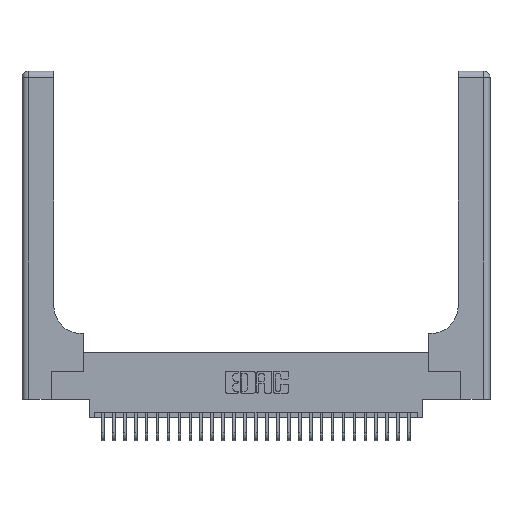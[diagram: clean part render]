
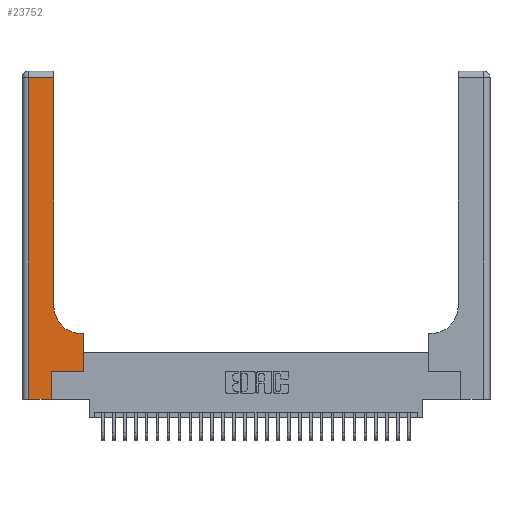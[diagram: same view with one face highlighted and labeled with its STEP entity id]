
A CAD part, top view. The second image highlights one B-rep face of the part: STEP entity #23752.
In plain terms, the highlighted planar face has unit normal (0, 0, 1).
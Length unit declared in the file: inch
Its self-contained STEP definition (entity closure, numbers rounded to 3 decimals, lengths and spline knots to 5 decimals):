
#189 = LINE ( 'NONE', #30230, #536 ) ;
#536 = VECTOR ( 'NONE', #6259, 39.37008 ) ;
#762 = VERTEX_POINT ( 'NONE', #8528 ) ;
#2404 = DIRECTION ( 'NONE',  ( -1., 0., 0. ) ) ;
#2814 = VERTEX_POINT ( 'NONE', #20282 ) ;
#2830 = VECTOR ( 'NONE', #19820, 39.37008 ) ;
#3628 = ORIENTED_EDGE ( 'NONE', *, *, #29415, .T. ) ;
#4681 = ORIENTED_EDGE ( 'NONE', *, *, #15141, .T. ) ;
#4830 = CARTESIAN_POINT ( 'NONE',  ( 0.2915, 2.94, 0.37 ) ) ;
#5075 = ORIENTED_EDGE ( 'NONE', *, *, #22319, .T. ) ;
#5270 = LINE ( 'NONE', #24816, #23941 ) ;
#5674 = DIRECTION ( 'NONE',  ( -1., 0., 0. ) ) ;
#5889 = DIRECTION ( 'NONE',  ( 0., 1., 0. ) ) ;
#6259 = DIRECTION ( 'NONE',  ( 1., 0., 0. ) ) ;
#6261 = VECTOR ( 'NONE', #5889, 39.37008 ) ;
#6720 = LINE ( 'NONE', #29518, #20437 ) ;
#7069 = EDGE_CURVE ( 'NONE', #27391, #20743, #17969, .T. ) ;
#7108 = CARTESIAN_POINT ( 'NONE',  ( 0.269, 0., 0.37 ) ) ;
#7911 = LINE ( 'NONE', #26861, #9107 ) ;
#8139 = LINE ( 'NONE', #10061, #2830 ) ;
#8460 = AXIS2_PLACEMENT_3D ( 'NONE', #17867, #22631, #10513 ) ;
#8528 = CARTESIAN_POINT ( 'NONE',  ( 0.5585, 0.6, 0.37 ) ) ;
#8895 = FACE_OUTER_BOUND ( 'NONE', #30482, .T. ) ;
#9107 = VECTOR ( 'NONE', #17098, 39.37008 ) ;
#10061 = CARTESIAN_POINT ( 'NONE',  ( 0.269, 0., 0.37 ) ) ;
#10513 = DIRECTION ( 'NONE',  ( -1., 0., 0. ) ) ;
#10747 = VERTEX_POINT ( 'NONE', #12897 ) ;
#10926 = EDGE_CURVE ( 'NONE', #20743, #25167, #189, .T. ) ;
#11225 = CIRCLE ( 'NONE', #23864, 0.25 ) ;
#12897 = CARTESIAN_POINT ( 'NONE',  ( 0.2915, 0.85, 0.37 ) ) ;
#13479 = CARTESIAN_POINT ( 'NONE',  ( 0.2915, 3., 0.37 ) ) ;
#13631 = ORIENTED_EDGE ( 'NONE', *, *, #23007, .T. ) ;
#15141 = EDGE_CURVE ( 'NONE', #29049, #27391, #6720, .T. ) ;
#17098 = DIRECTION ( 'NONE',  ( 1., 0., 0. ) ) ;
#17388 = EDGE_CURVE ( 'NONE', #25256, #10747, #11225, .T. ) ;
#17631 = CARTESIAN_POINT ( 'NONE',  ( 0.06, 0., 0.37 ) ) ;
#17685 = LINE ( 'NONE', #27494, #6261 ) ;
#17867 = CARTESIAN_POINT ( 'NONE',  ( 0., 3., 0.37 ) ) ;
#17969 = LINE ( 'NONE', #26387, #27877 ) ;
#19075 = LINE ( 'NONE', #13479, #24758 ) ;
#19247 = CARTESIAN_POINT ( 'NONE',  ( 0.5415, 0.6, 0.37 ) ) ;
#19820 = DIRECTION ( 'NONE',  ( 0., 1., 0. ) ) ;
#20163 = ORIENTED_EDGE ( 'NONE', *, *, #17388, .T. ) ;
#20282 = CARTESIAN_POINT ( 'NONE',  ( 0.269, 0.25, 0.37 ) ) ;
#20437 = VECTOR ( 'NONE', #2404, 39.37008 ) ;
#20743 = VERTEX_POINT ( 'NONE', #17631 ) ;
#21240 = EDGE_CURVE ( 'NONE', #762, #25256, #5270, .T. ) ;
#22319 = EDGE_CURVE ( 'NONE', #25167, #2814, #8139, .T. ) ;
#22626 = ORIENTED_EDGE ( 'NONE', *, *, #21240, .T. ) ;
#22631 = DIRECTION ( 'NONE',  ( 0., 0., -1. ) ) ;
#23007 = EDGE_CURVE ( 'NONE', #26993, #762, #17685, .T. ) ;
#23752 = ADVANCED_FACE ( 'NONE', ( #8895 ), #30324, .F. ) ;
#23864 = AXIS2_PLACEMENT_3D ( 'NONE', #25898, #26003, #28340 ) ;
#23941 = VECTOR ( 'NONE', #5674, 39.37008 ) ;
#24340 = DIRECTION ( 'NONE',  ( 0., -1., 0. ) ) ;
#24758 = VECTOR ( 'NONE', #25802, 39.37008 ) ;
#24816 = CARTESIAN_POINT ( 'NONE',  ( 0.2915, 0.6, 0.37 ) ) ;
#25167 = VERTEX_POINT ( 'NONE', #7108 ) ;
#25256 = VERTEX_POINT ( 'NONE', #19247 ) ;
#25802 = DIRECTION ( 'NONE',  ( 0., 1., 0. ) ) ;
#25898 = CARTESIAN_POINT ( 'NONE',  ( 0.5415, 0.85, 0.37 ) ) ;
#25984 = ORIENTED_EDGE ( 'NONE', *, *, #10926, .T. ) ;
#26003 = DIRECTION ( 'NONE',  ( 0., 0., -1. ) ) ;
#26038 = EDGE_CURVE ( 'NONE', #2814, #26993, #7911, .T. ) ;
#26157 = ORIENTED_EDGE ( 'NONE', *, *, #26038, .T. ) ;
#26387 = CARTESIAN_POINT ( 'NONE',  ( 0.06, 3., 0.37 ) ) ;
#26861 = CARTESIAN_POINT ( 'NONE',  ( 0.269, 0.25, 0.37 ) ) ;
#26993 = VERTEX_POINT ( 'NONE', #30573 ) ;
#27391 = VERTEX_POINT ( 'NONE', #27665 ) ;
#27494 = CARTESIAN_POINT ( 'NONE',  ( 0.5585, 0.25, 0.37 ) ) ;
#27665 = CARTESIAN_POINT ( 'NONE',  ( 0.06, 2.94, 0.37 ) ) ;
#27877 = VECTOR ( 'NONE', #24340, 39.37008 ) ;
#28340 = DIRECTION ( 'NONE',  ( 1., 0., 0. ) ) ;
#29049 = VERTEX_POINT ( 'NONE', #4830 ) ;
#29415 = EDGE_CURVE ( 'NONE', #10747, #29049, #19075, .T. ) ;
#29498 = ORIENTED_EDGE ( 'NONE', *, *, #7069, .T. ) ;
#29518 = CARTESIAN_POINT ( 'NONE',  ( 0., 2.94, 0.37 ) ) ;
#30230 = CARTESIAN_POINT ( 'NONE',  ( 0., 0., 0.37 ) ) ;
#30324 = PLANE ( 'NONE',  #8460 ) ;
#30482 = EDGE_LOOP ( 'NONE', ( #3628, #4681, #29498, #25984, #5075, #26157, #13631, #22626, #20163 ) ) ;
#30573 = CARTESIAN_POINT ( 'NONE',  ( 0.5585, 0.25, 0.37 ) ) ;
